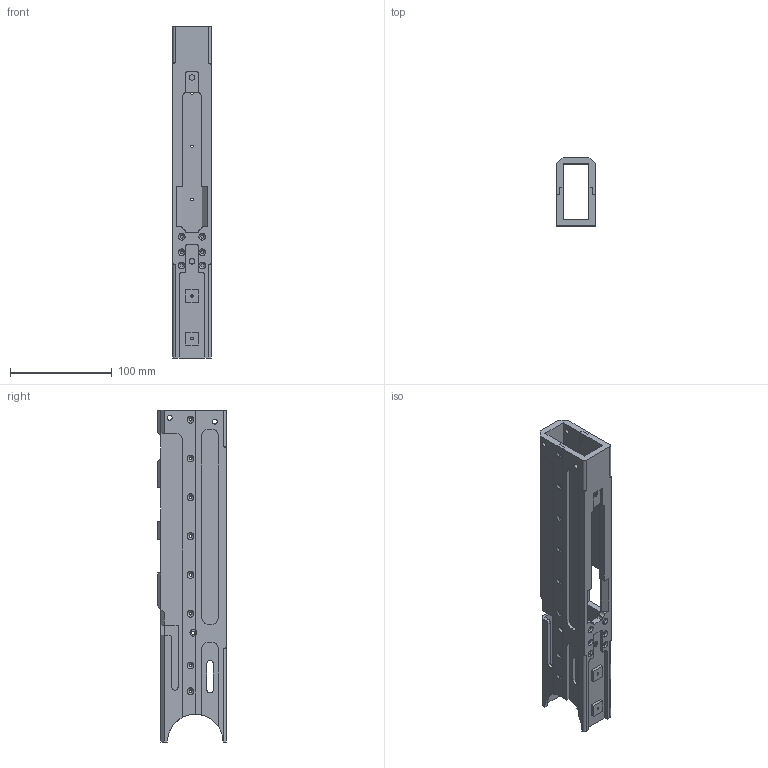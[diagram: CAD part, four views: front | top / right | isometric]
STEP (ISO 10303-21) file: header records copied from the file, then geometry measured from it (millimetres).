
FILE_DESCRIPTION (( 'STEP AP214' ), '1' );
FILE_NAME ('PPDW9 V4 Split Upper.STEP', '2020-12-31T17:57:19', ( '' ), ( '' ), 'SwSTEP 2.0', 'SolidWorks 2020', '' );
FILE_SCHEMA (( 'AUTOMOTIVE_DESIGN' ));
Length unit declared in the file: inch
Products named in the file (3): PPDW9 V4 split upper bottom; PPDW9 V4 split upper top; PPDW9 V4 Split Upper
Assembly tree (2 placements, depth 2):
  PPDW9 V4 Split Upper
    PPDW9 V4 split upper bottom
    PPDW9 V4 split upper top
Bounding box: 38.1 x 67.31 x 325.95 mm (x, y, z)
Volume: 234484.5 mm3; surface area: 132487.9 mm2
Topology: 2 solids, 2 shells, 366 faces, 1001 edges, 632 vertices
Faces by surface type: cylinder 166, plane 140, cone 48, bspline 8, torus 4
Entity records: 12661 total; most frequent: CARTESIAN_POINT 2264, DIRECTION 2087, ORIENTED_EDGE 1986, EDGE_CURVE 993, AXIS2_PLACEMENT_3D 751, VERTEX_POINT 632, LINE 585, VECTOR 585
